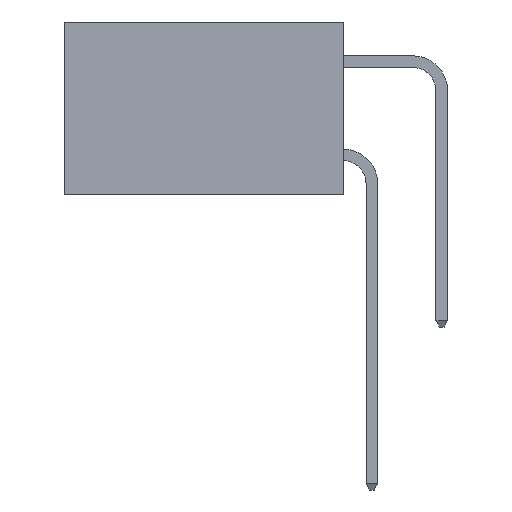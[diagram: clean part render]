
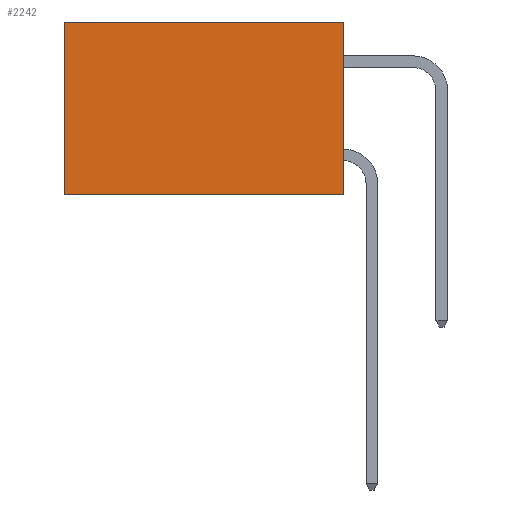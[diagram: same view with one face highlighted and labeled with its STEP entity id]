
A CAD part, left-side view. The second image highlights one B-rep face of the part: STEP entity #2242.
In plain terms, the highlighted planar face has unit normal (-1, 0, 0).
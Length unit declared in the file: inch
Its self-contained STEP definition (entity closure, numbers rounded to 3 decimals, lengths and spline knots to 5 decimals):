
#574 = CARTESIAN_POINT ( 'NONE',  ( 0.2615, 0., 0. ) ) ;
#586 = ORIENTED_EDGE ( 'NONE', *, *, #8083, .T. ) ;
#1091 = VERTEX_POINT ( 'NONE', #10197 ) ;
#1194 = VERTEX_POINT ( 'NONE', #3821 ) ;
#2204 = DIRECTION ( 'NONE',  ( 1., 0., 0. ) ) ;
#2242 = ADVANCED_FACE ( 'NONE', ( #4680 ), #14352, .F. ) ;
#3284 = CARTESIAN_POINT ( 'NONE',  ( 0.2615, 0.6, -0.37 ) ) ;
#3300 = EDGE_CURVE ( 'NONE', #1091, #10884, #10162, .T. ) ;
#3493 = LINE ( 'NONE', #574, #13411 ) ;
#3821 = CARTESIAN_POINT ( 'NONE',  ( 0.2615, 0.6, 0. ) ) ;
#3887 = DIRECTION ( 'NONE',  ( 0., 0., -1. ) ) ;
#3964 = EDGE_CURVE ( 'NONE', #1194, #10884, #17787, .T. ) ;
#4280 = AXIS2_PLACEMENT_3D ( 'NONE', #13836, #2204, #3887 ) ;
#4680 = FACE_OUTER_BOUND ( 'NONE', #15171, .T. ) ;
#7470 = EDGE_CURVE ( 'NONE', #15969, #1091, #16910, .T. ) ;
#7654 = DIRECTION ( 'NONE',  ( 0., 0., -1. ) ) ;
#7999 = CARTESIAN_POINT ( 'NONE',  ( 0.2615, 0., -0.37 ) ) ;
#8083 = EDGE_CURVE ( 'NONE', #15969, #1194, #3493, .T. ) ;
#9171 = ORIENTED_EDGE ( 'NONE', *, *, #3964, .T. ) ;
#10162 = LINE ( 'NONE', #11255, #14347 ) ;
#10197 = CARTESIAN_POINT ( 'NONE',  ( 0.2615, 0., -0.37 ) ) ;
#10356 = VECTOR ( 'NONE', #10679, 39.37008 ) ;
#10679 = DIRECTION ( 'NONE',  ( 0., 0., -1. ) ) ;
#10884 = VERTEX_POINT ( 'NONE', #3284 ) ;
#11195 = DIRECTION ( 'NONE',  ( 0., 1., 0. ) ) ;
#11255 = CARTESIAN_POINT ( 'NONE',  ( 0.2615, 0., -0.37 ) ) ;
#11756 = CARTESIAN_POINT ( 'NONE',  ( 0.2615, 0.6, -0.37 ) ) ;
#12769 = VECTOR ( 'NONE', #7654, 39.37008 ) ;
#13411 = VECTOR ( 'NONE', #17965, 39.37008 ) ;
#13836 = CARTESIAN_POINT ( 'NONE',  ( 0.2615, 0., -0.37 ) ) ;
#14347 = VECTOR ( 'NONE', #11195, 39.37008 ) ;
#14352 = PLANE ( 'NONE',  #4280 ) ;
#15171 = EDGE_LOOP ( 'NONE', ( #9171, #15276, #17765, #586 ) ) ;
#15276 = ORIENTED_EDGE ( 'NONE', *, *, #3300, .F. ) ;
#15969 = VERTEX_POINT ( 'NONE', #17613 ) ;
#16910 = LINE ( 'NONE', #7999, #12769 ) ;
#17613 = CARTESIAN_POINT ( 'NONE',  ( 0.2615, 0., 0. ) ) ;
#17765 = ORIENTED_EDGE ( 'NONE', *, *, #7470, .F. ) ;
#17787 = LINE ( 'NONE', #11756, #10356 ) ;
#17965 = DIRECTION ( 'NONE',  ( 0., 1., 0. ) ) ;
